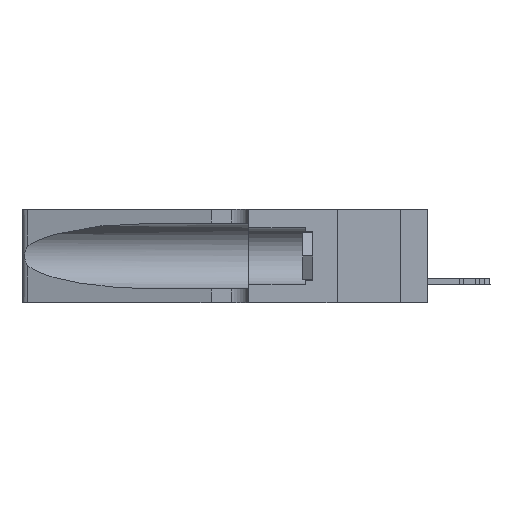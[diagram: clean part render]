
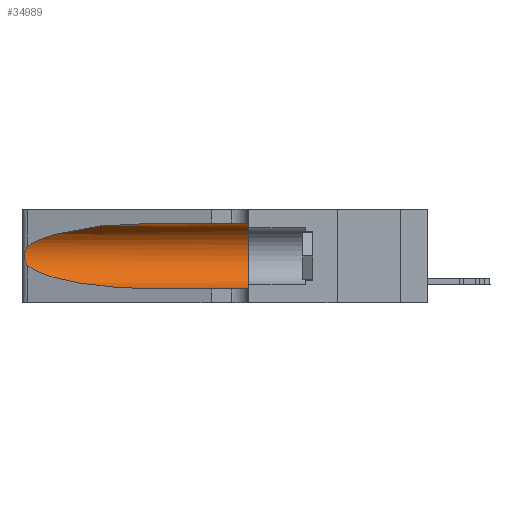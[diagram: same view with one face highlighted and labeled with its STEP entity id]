
A CAD part, left-side view. The second image highlights one B-rep face of the part: STEP entity #34989.
In plain terms, the highlighted cylindrical face has radius 3.308 mm (diameter 6.617 mm), a partial arc.
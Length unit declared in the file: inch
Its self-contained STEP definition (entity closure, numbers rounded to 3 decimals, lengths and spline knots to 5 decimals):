
#1339 = ORIENTED_EDGE ( 'NONE', *, *, #13875, .T. ) ;
#1384 = CARTESIAN_POINT ( 'NONE',  ( 0.25787, 1.23484, 0.2124 ) ) ;
#1642 = VERTEX_POINT ( 'NONE', #46861 ) ;
#1776 = CARTESIAN_POINT ( 'NONE',  ( 0.25856, 1.23593, 0.16098 ) ) ;
#2799 = CARTESIAN_POINT ( 'NONE',  ( 0.1305, 0.35, 0.05475 ) ) ;
#4501 = ORIENTED_EDGE ( 'NONE', *, *, #22905, .T. ) ;
#6999 = VERTEX_POINT ( 'NONE', #42890 ) ;
#7214 = CIRCLE ( 'NONE', #23334, 0.13025 ) ;
#7365 = CARTESIAN_POINT ( 'NONE',  ( 0.1305, 0.72297, 0.05475 ) ) ;
#8091 = VERTEX_POINT ( 'NONE', #10513 ) ;
#8157 = VECTOR ( 'NONE', #46032, 39.37008 ) ;
#8245 = ORIENTED_EDGE ( 'NONE', *, *, #27221, .T. ) ;
#8797 = DIRECTION ( 'NONE',  ( 0., 0., -1. ) ) ;
#9739 = CARTESIAN_POINT ( 'NONE',  ( 0.25639, 1.23184, 0.21858 ) ) ;
#10513 = CARTESIAN_POINT ( 'NONE',  ( 0.25487, 1.22718, 0.22369 ) ) ;
#11423 = AXIS2_PLACEMENT_3D ( 'NONE', #32166, #44606, #8797 ) ;
#12395 = ORIENTED_EDGE ( 'NONE', *, *, #18106, .T. ) ;
#13875 = EDGE_CURVE ( 'NONE', #6999, #15082, #38653, .T. ) ;
#14766 = DIRECTION ( 'NONE',  ( 0., 0., 1. ) ) ;
#14801 = EDGE_LOOP ( 'NONE', ( #8245, #12395, #4501, #1339, #24188, #35913 ) ) ;
#15082 = VERTEX_POINT ( 'NONE', #2799 ) ;
#17201 = EDGE_CURVE ( 'NONE', #50290, #1642, #46254, .T. ) ;
#17777 = CARTESIAN_POINT ( 'NONE',  ( 0.26075, 1.23896, 0.19203 ) ) ;
#18106 = EDGE_CURVE ( 'NONE', #8091, #40650, #40409, .T. ) ;
#21780 = CARTESIAN_POINT ( 'NONE',  ( 0.26017, 1.23833, 0.17102 ) ) ;
#22905 = EDGE_CURVE ( 'NONE', #40650, #6999, #29047, .T. ) ;
#22983 = CYLINDRICAL_SURFACE ( 'NONE', #11423, 0.13025 ) ;
#23334 = AXIS2_PLACEMENT_3D ( 'NONE', #38139, #46527, #14766 ) ;
#24188 = ORIENTED_EDGE ( 'NONE', *, *, #43062, .F. ) ;
#25464 = CARTESIAN_POINT ( 'NONE',  ( 0.25555, 1.22994, 0.2215 ) ) ;
#25825 = CARTESIAN_POINT ( 'NONE',  ( 0.25639, 1.23186, 0.15144 ) ) ;
#26025 = FACE_OUTER_BOUND ( 'NONE', #14801, .T. ) ;
#26289 = CARTESIAN_POINT ( 'NONE',  ( 0.25487, 1.22718, 0.14631 ) ) ;
#26380 = CARTESIAN_POINT ( 'NONE',  ( 0.25487, 1.22718, 0.14631 ) ) ;
#27221 = EDGE_CURVE ( 'NONE', #50290, #8091, #33566, .T. ) ;
#29047 =( BOUNDED_CURVE ( )  B_SPLINE_CURVE ( 3, ( #39007, #31358, #34983, #7365 ),
 .UNSPECIFIED., .F., .F. ) 
 B_SPLINE_CURVE_WITH_KNOTS ( ( 4, 4 ),
 ( 3.44316, 4.71239 ),
 .UNSPECIFIED. ) 
 CURVE ( )  GEOMETRIC_REPRESENTATION_ITEM ( )  RATIONAL_B_SPLINE_CURVE ( ( 1., 0.87, 0.87, 1. ) ) 
 REPRESENTATION_ITEM ( '' )  );
#29490 = CARTESIAN_POINT ( 'NONE',  ( 0.25854, 1.2359, 0.20912 ) ) ;
#29622 = CARTESIAN_POINT ( 'NONE',  ( 0.1305, 1.61858, 0.31525 ) ) ;
#31358 = CARTESIAN_POINT ( 'NONE',  ( 0.2373, 1.15595, 0.08982 ) ) ;
#32166 = CARTESIAN_POINT ( 'NONE',  ( 0.1305, 1.61858, 0.185 ) ) ;
#32499 = CARTESIAN_POINT ( 'NONE',  ( 0.1305, 0.72297, 0.31525 ) ) ;
#33566 =( BOUNDED_CURVE ( )  B_SPLINE_CURVE ( 3, ( #46708, #42177, #42552, #50162 ),
 .UNSPECIFIED., .F., .F. ) 
 B_SPLINE_CURVE_WITH_KNOTS ( ( 4, 4 ),
 ( 1.5708, 2.84003 ),
 .UNSPECIFIED. ) 
 CURVE ( )  GEOMETRIC_REPRESENTATION_ITEM ( )  RATIONAL_B_SPLINE_CURVE ( ( 1., 0.87, 0.87, 1. ) ) 
 REPRESENTATION_ITEM ( '' )  );
#34912 = VECTOR ( 'NONE', #35882, 39.37008 ) ;
#34983 = CARTESIAN_POINT ( 'NONE',  ( 0.18966, 0.96281, 0.05475 ) ) ;
#34989 = ADVANCED_FACE ( 'NONE', ( #26025 ), #22983, .F. ) ;
#35724 = CARTESIAN_POINT ( 'NONE',  ( 0.1305, 1.61858, 0.05475 ) ) ;
#35882 = DIRECTION ( 'NONE',  ( 0., -1., 0. ) ) ;
#35913 = ORIENTED_EDGE ( 'NONE', *, *, #17201, .F. ) ;
#38139 = CARTESIAN_POINT ( 'NONE',  ( 0.1305, 0.35, 0.185 ) ) ;
#38653 = LINE ( 'NONE', #35724, #34912 ) ;
#39007 = CARTESIAN_POINT ( 'NONE',  ( 0.25487, 1.22718, 0.14631 ) ) ;
#40409 = B_SPLINE_CURVE_WITH_KNOTS ( 'NONE', 3,
 ( #49333, #25464, #9739, #1384, #29490, #41706, #17777, #45686, #21780, #1776, #49676, #25825, #42830, #26380 ),
 .UNSPECIFIED., .F., .F.,
 ( 4, 2, 2, 2, 2, 2, 4 ),
 ( 0., 0.00027, 0.00053, 0.00107, 0.0016, 0.00187, 0.00214 ),
 .UNSPECIFIED. ) ;
#40650 = VERTEX_POINT ( 'NONE', #26289 ) ;
#41706 = CARTESIAN_POINT ( 'NONE',  ( 0.26018, 1.23835, 0.19895 ) ) ;
#42177 = CARTESIAN_POINT ( 'NONE',  ( 0.18966, 0.96281, 0.31525 ) ) ;
#42552 = CARTESIAN_POINT ( 'NONE',  ( 0.2373, 1.15595, 0.28018 ) ) ;
#42830 = CARTESIAN_POINT ( 'NONE',  ( 0.25555, 1.22993, 0.14849 ) ) ;
#42890 = CARTESIAN_POINT ( 'NONE',  ( 0.1305, 0.72297, 0.05475 ) ) ;
#43062 = EDGE_CURVE ( 'NONE', #1642, #15082, #7214, .T. ) ;
#44606 = DIRECTION ( 'NONE',  ( 0., -1., 0. ) ) ;
#45686 = CARTESIAN_POINT ( 'NONE',  ( 0.26075, 1.23896, 0.178 ) ) ;
#46032 = DIRECTION ( 'NONE',  ( 0., -1., 0. ) ) ;
#46254 = LINE ( 'NONE', #29622, #8157 ) ;
#46527 = DIRECTION ( 'NONE',  ( 0., 1., 0. ) ) ;
#46708 = CARTESIAN_POINT ( 'NONE',  ( 0.1305, 0.72297, 0.31525 ) ) ;
#46861 = CARTESIAN_POINT ( 'NONE',  ( 0.1305, 0.35, 0.31525 ) ) ;
#49333 = CARTESIAN_POINT ( 'NONE',  ( 0.25487, 1.22718, 0.22369 ) ) ;
#49676 = CARTESIAN_POINT ( 'NONE',  ( 0.25789, 1.23486, 0.15765 ) ) ;
#50162 = CARTESIAN_POINT ( 'NONE',  ( 0.25487, 1.22718, 0.22369 ) ) ;
#50290 = VERTEX_POINT ( 'NONE', #32499 ) ;
